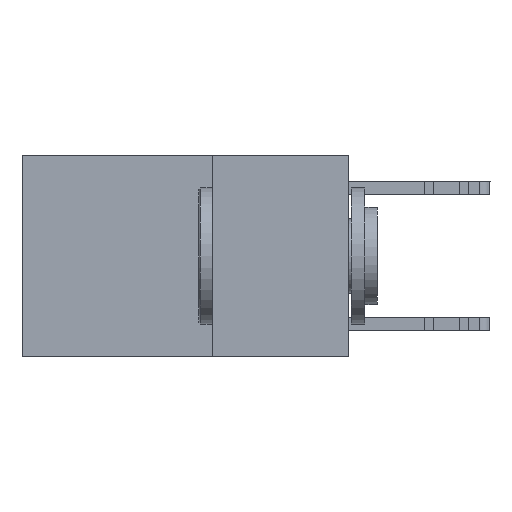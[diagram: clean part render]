
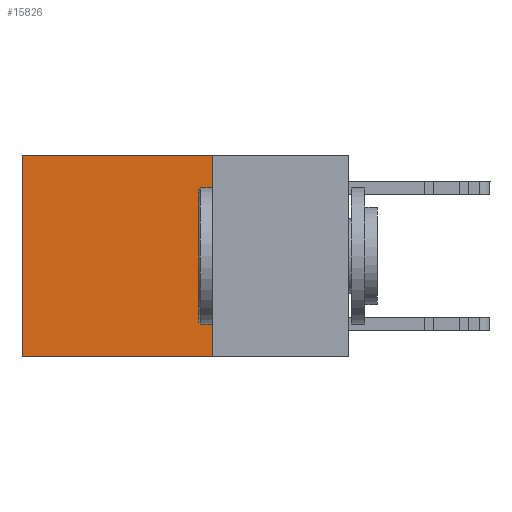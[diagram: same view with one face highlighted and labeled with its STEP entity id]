
A CAD part, left-side view. The second image highlights one B-rep face of the part: STEP entity #15826.
In plain terms, the highlighted planar face has unit normal (-1, 0, 0).
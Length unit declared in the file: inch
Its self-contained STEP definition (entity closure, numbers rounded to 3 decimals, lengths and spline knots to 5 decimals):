
#1101 = VERTEX_POINT ( 'NONE', #5427 ) ;
#1993 = LINE ( 'NONE', #11450, #23792 ) ;
#2175 = EDGE_LOOP ( 'NONE', ( #20947, #27284, #12547, #7893 ) ) ;
#3088 = VECTOR ( 'NONE', #15679, 39.37008 ) ;
#3889 = EDGE_CURVE ( 'NONE', #22762, #1101, #11030, .T. ) ;
#5427 = CARTESIAN_POINT ( 'NONE',  ( 0.2625, 0.6, -0.37 ) ) ;
#5697 = DIRECTION ( 'NONE',  ( 1., 0., 0. ) ) ;
#6172 = EDGE_CURVE ( 'NONE', #16455, #13243, #15371, .T. ) ;
#7207 = DIRECTION ( 'NONE',  ( 0., 0., -1. ) ) ;
#7332 = DIRECTION ( 'NONE',  ( 0., 0., -1. ) ) ;
#7893 = ORIENTED_EDGE ( 'NONE', *, *, #6172, .T. ) ;
#8059 = PLANE ( 'NONE',  #8415 ) ;
#8415 = AXIS2_PLACEMENT_3D ( 'NONE', #27233, #5697, #7207 ) ;
#8440 = CARTESIAN_POINT ( 'NONE',  ( 0.2625, 0.25, 0. ) ) ;
#9778 = VECTOR ( 'NONE', #19111, 39.37008 ) ;
#11030 = LINE ( 'NONE', #27834, #28919 ) ;
#11450 = CARTESIAN_POINT ( 'NONE',  ( 0.2625, 0.6, 0. ) ) ;
#12547 = ORIENTED_EDGE ( 'NONE', *, *, #27932, .F. ) ;
#13243 = VERTEX_POINT ( 'NONE', #21641 ) ;
#15371 = LINE ( 'NONE', #8440, #3088 ) ;
#15544 = CARTESIAN_POINT ( 'NONE',  ( 0.2625, 0.25, 0. ) ) ;
#15679 = DIRECTION ( 'NONE',  ( 0., 1., 0. ) ) ;
#15826 = ADVANCED_FACE ( 'NONE', ( #29598 ), #8059, .F. ) ;
#16455 = VERTEX_POINT ( 'NONE', #15544 ) ;
#19111 = DIRECTION ( 'NONE',  ( 0., 0., -1. ) ) ;
#19267 = LINE ( 'NONE', #30910, #9778 ) ;
#20883 = DIRECTION ( 'NONE',  ( 0., 1., 0. ) ) ;
#20947 = ORIENTED_EDGE ( 'NONE', *, *, #27944, .T. ) ;
#21641 = CARTESIAN_POINT ( 'NONE',  ( 0.2625, 0.6, 0. ) ) ;
#22762 = VERTEX_POINT ( 'NONE', #29206 ) ;
#23792 = VECTOR ( 'NONE', #7332, 39.37008 ) ;
#27233 = CARTESIAN_POINT ( 'NONE',  ( 0.2625, 0.25, 0. ) ) ;
#27284 = ORIENTED_EDGE ( 'NONE', *, *, #3889, .F. ) ;
#27834 = CARTESIAN_POINT ( 'NONE',  ( 0.2625, 0.25, -0.37 ) ) ;
#27932 = EDGE_CURVE ( 'NONE', #16455, #22762, #19267, .T. ) ;
#27944 = EDGE_CURVE ( 'NONE', #13243, #1101, #1993, .T. ) ;
#28919 = VECTOR ( 'NONE', #20883, 39.37008 ) ;
#29206 = CARTESIAN_POINT ( 'NONE',  ( 0.2625, 0.25, -0.37 ) ) ;
#29598 = FACE_OUTER_BOUND ( 'NONE', #2175, .T. ) ;
#30910 = CARTESIAN_POINT ( 'NONE',  ( 0.2625, 0.25, 0. ) ) ;
